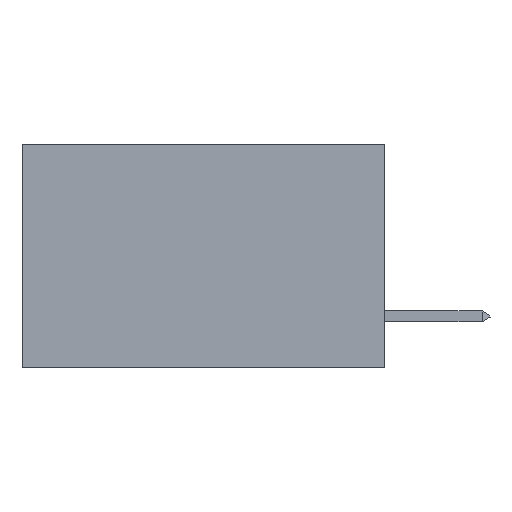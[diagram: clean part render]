
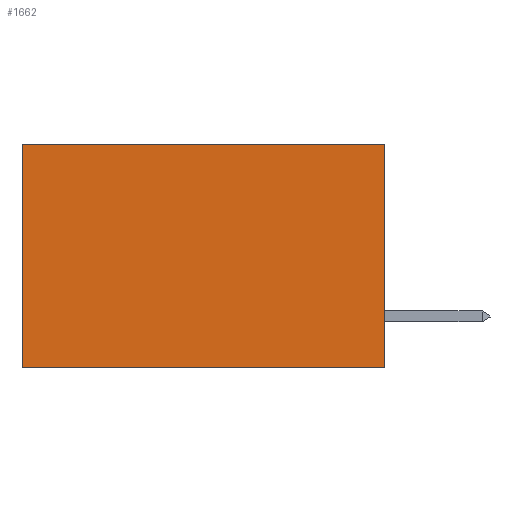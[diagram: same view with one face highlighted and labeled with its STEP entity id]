
A CAD part, left-side view. The second image highlights one B-rep face of the part: STEP entity #1662.
In plain terms, the highlighted planar face has unit normal (-1, 0, 0).
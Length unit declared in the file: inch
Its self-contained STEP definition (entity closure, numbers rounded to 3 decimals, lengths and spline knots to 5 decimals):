
#1662 = ADVANCED_FACE ( 'NONE', ( #5892 ), #16612, .F. ) ;
#3347 = CARTESIAN_POINT ( 'NONE',  ( 0.2875, 0., 0. ) ) ;
#3679 = ORIENTED_EDGE ( 'NONE', *, *, #25156, .F. ) ;
#4250 = VERTEX_POINT ( 'NONE', #6775 ) ;
#5477 = CARTESIAN_POINT ( 'NONE',  ( 0.2875, 0.6, -0.37 ) ) ;
#5503 = DIRECTION ( 'NONE',  ( 1., 0., 0. ) ) ;
#5724 = ORIENTED_EDGE ( 'NONE', *, *, #15893, .F. ) ;
#5892 = FACE_OUTER_BOUND ( 'NONE', #23961, .T. ) ;
#6775 = CARTESIAN_POINT ( 'NONE',  ( 0.2875, 0., 0. ) ) ;
#7481 = LINE ( 'NONE', #24435, #11696 ) ;
#7749 = LINE ( 'NONE', #9776, #20285 ) ;
#8850 = DIRECTION ( 'NONE',  ( 0., 1., 0. ) ) ;
#9670 = CARTESIAN_POINT ( 'NONE',  ( 0.2875, 0., -0.37 ) ) ;
#9695 = LINE ( 'NONE', #14100, #14938 ) ;
#9776 = CARTESIAN_POINT ( 'NONE',  ( 0.2875, 0.6, 0. ) ) ;
#10259 = CARTESIAN_POINT ( 'NONE',  ( 0.2875, 0., -0.37 ) ) ;
#11696 = VECTOR ( 'NONE', #20083, 39.37008 ) ;
#11992 = DIRECTION ( 'NONE',  ( 0., 0., -1. ) ) ;
#12739 = ORIENTED_EDGE ( 'NONE', *, *, #16404, .T. ) ;
#14056 = VERTEX_POINT ( 'NONE', #26310 ) ;
#14100 = CARTESIAN_POINT ( 'NONE',  ( 0.2875, 0., 0. ) ) ;
#14226 = VERTEX_POINT ( 'NONE', #5477 ) ;
#14235 = AXIS2_PLACEMENT_3D ( 'NONE', #3347, #5503, #25701 ) ;
#14747 = DIRECTION ( 'NONE',  ( 0., 1., 0. ) ) ;
#14938 = VECTOR ( 'NONE', #8850, 39.37008 ) ;
#15893 = EDGE_CURVE ( 'NONE', #23014, #14226, #26906, .T. ) ;
#16404 = EDGE_CURVE ( 'NONE', #4250, #14056, #9695, .T. ) ;
#16612 = PLANE ( 'NONE',  #14235 ) ;
#20083 = DIRECTION ( 'NONE',  ( 0., 0., -1. ) ) ;
#20285 = VECTOR ( 'NONE', #11992, 39.37008 ) ;
#20604 = EDGE_CURVE ( 'NONE', #14056, #14226, #7749, .T. ) ;
#23014 = VERTEX_POINT ( 'NONE', #10259 ) ;
#23041 = ORIENTED_EDGE ( 'NONE', *, *, #20604, .T. ) ;
#23961 = EDGE_LOOP ( 'NONE', ( #23041, #5724, #3679, #12739 ) ) ;
#24435 = CARTESIAN_POINT ( 'NONE',  ( 0.2875, 0., 0. ) ) ;
#25054 = VECTOR ( 'NONE', #14747, 39.37008 ) ;
#25156 = EDGE_CURVE ( 'NONE', #4250, #23014, #7481, .T. ) ;
#25701 = DIRECTION ( 'NONE',  ( 0., 0., -1. ) ) ;
#26310 = CARTESIAN_POINT ( 'NONE',  ( 0.2875, 0.6, 0. ) ) ;
#26906 = LINE ( 'NONE', #9670, #25054 ) ;
